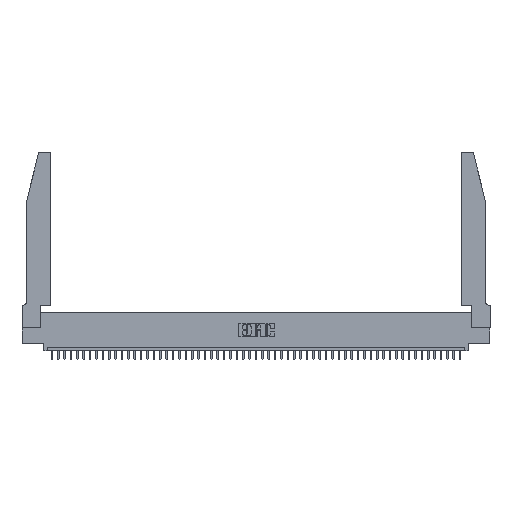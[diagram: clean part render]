
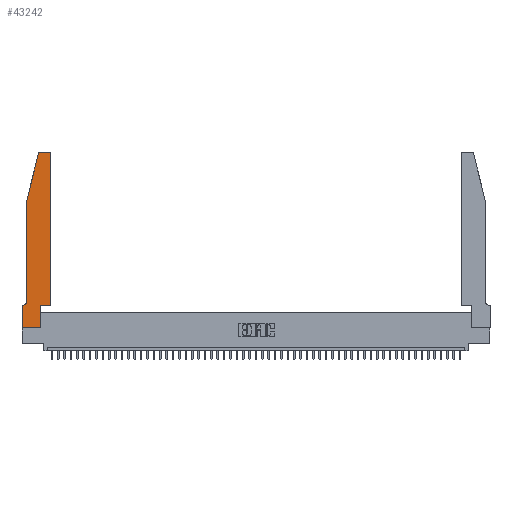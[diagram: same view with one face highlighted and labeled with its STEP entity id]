
A CAD part, top view. The second image highlights one B-rep face of the part: STEP entity #43242.
In plain terms, the highlighted planar face has unit normal (0, 0, 1).
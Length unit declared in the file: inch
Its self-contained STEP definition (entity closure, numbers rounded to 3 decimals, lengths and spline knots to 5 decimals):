
#495 = EDGE_CURVE ( 'NONE', #29341, #40950, #36946, .T. ) ;
#590 = EDGE_CURVE ( 'NONE', #809, #47112, #31429, .T. ) ;
#809 = VERTEX_POINT ( 'NONE', #6096 ) ;
#1147 = ORIENTED_EDGE ( 'NONE', *, *, #14008, .T. ) ;
#1455 = CARTESIAN_POINT ( 'NONE',  ( 0.0755, 0.35, 0.37 ) ) ;
#1528 = DIRECTION ( 'NONE',  ( -0.239, -0.971, 0. ) ) ;
#2582 = EDGE_CURVE ( 'NONE', #37422, #9412, #15421, .T. ) ;
#3336 = VERTEX_POINT ( 'NONE', #26846 ) ;
#4393 = CARTESIAN_POINT ( 'NONE',  ( 0.2865, 0.35, 0.37 ) ) ;
#5661 = CARTESIAN_POINT ( 'NONE',  ( 0.4205, 2.75, 0.37 ) ) ;
#5917 = CARTESIAN_POINT ( 'NONE',  ( 0.0055, 0.42, 0.37 ) ) ;
#6055 = DIRECTION ( 'NONE',  ( 0., 1., 0. ) ) ;
#6062 = LINE ( 'NONE', #7796, #25618 ) ;
#6096 = CARTESIAN_POINT ( 'NONE',  ( 0., 0., 0.37 ) ) ;
#7111 = EDGE_CURVE ( 'NONE', #3336, #15386, #10087, .T. ) ;
#7328 = ORIENTED_EDGE ( 'NONE', *, *, #14527, .T. ) ;
#7796 = CARTESIAN_POINT ( 'NONE',  ( 0.0755, 2., 0.37 ) ) ;
#8619 = ORIENTED_EDGE ( 'NONE', *, *, #26098, .T. ) ;
#8633 = PLANE ( 'NONE',  #12417 ) ;
#8872 = EDGE_CURVE ( 'NONE', #28863, #3336, #14033, .T. ) ;
#9007 = CARTESIAN_POINT ( 'NONE',  ( 0.4505, 0.35, 0.37 ) ) ;
#9250 = CIRCLE ( 'NONE', #36645, 0.03 ) ;
#9412 = VERTEX_POINT ( 'NONE', #22012 ) ;
#9848 = LINE ( 'NONE', #14392, #38137 ) ;
#9926 = VECTOR ( 'NONE', #36246, 39.37008 ) ;
#10087 = LINE ( 'NONE', #1455, #43846 ) ;
#11253 = DIRECTION ( 'NONE',  ( -1., 0., 0. ) ) ;
#11617 = DIRECTION ( 'NONE',  ( 1., 0., 0. ) ) ;
#11722 = VECTOR ( 'NONE', #1528, 39.37008 ) ;
#12343 = CIRCLE ( 'NONE', #21338, 0.03 ) ;
#12417 = AXIS2_PLACEMENT_3D ( 'NONE', #43455, #39219, #27490 ) ;
#13644 = EDGE_LOOP ( 'NONE', ( #7328, #49788, #37981, #8619, #37603, #48572, #25549, #42449, #34405, #46045, #41662, #1147 ) ) ;
#13886 = DIRECTION ( 'NONE',  ( 1., 0., 0. ) ) ;
#14008 = EDGE_CURVE ( 'NONE', #40950, #33710, #9250, .T. ) ;
#14033 = CIRCLE ( 'NONE', #16142, 0.07 ) ;
#14392 = CARTESIAN_POINT ( 'NONE',  ( 0.2865, 0.35, 0.37 ) ) ;
#14524 = DIRECTION ( 'NONE',  ( 0., -1., 0. ) ) ;
#14527 = EDGE_CURVE ( 'NONE', #33710, #45415, #20190, .T. ) ;
#15218 = CARTESIAN_POINT ( 'NONE',  ( 0.2605, 2.75, 0.37 ) ) ;
#15386 = VERTEX_POINT ( 'NONE', #41756 ) ;
#15421 = LINE ( 'NONE', #40391, #11722 ) ;
#16142 = AXIS2_PLACEMENT_3D ( 'NONE', #5917, #32952, #17025 ) ;
#17025 = DIRECTION ( 'NONE',  ( -1., 0., 0. ) ) ;
#18484 = CARTESIAN_POINT ( 'NONE',  ( 0., 0., 0.37 ) ) ;
#20190 = LINE ( 'NONE', #15218, #36044 ) ;
#20630 = DIRECTION ( 'NONE',  ( 0., 1., 0. ) ) ;
#20795 = CARTESIAN_POINT ( 'NONE',  ( 0.4505, 0.35, 0.37 ) ) ;
#21338 = AXIS2_PLACEMENT_3D ( 'NONE', #27720, #23126, #11617 ) ;
#22012 = CARTESIAN_POINT ( 'NONE',  ( 0.0755, 2., 0.37 ) ) ;
#22039 = DIRECTION ( 'NONE',  ( 1., 0., 0. ) ) ;
#23126 = DIRECTION ( 'NONE',  ( 0., 0., 1. ) ) ;
#24107 = VECTOR ( 'NONE', #14524, 39.37008 ) ;
#24660 = VECTOR ( 'NONE', #20630, 39.37008 ) ;
#25549 = ORIENTED_EDGE ( 'NONE', *, *, #44406, .T. ) ;
#25618 = VECTOR ( 'NONE', #35502, 39.37008 ) ;
#26098 = EDGE_CURVE ( 'NONE', #9412, #28863, #6062, .T. ) ;
#26796 = CARTESIAN_POINT ( 'NONE',  ( 0.4505, 2.72, 0.37 ) ) ;
#26846 = CARTESIAN_POINT ( 'NONE',  ( 0.0055, 0.35, 0.37 ) ) ;
#27490 = DIRECTION ( 'NONE',  ( 1., 0., 0. ) ) ;
#27720 = CARTESIAN_POINT ( 'NONE',  ( 0.284, 2.72, 0.37 ) ) ;
#28027 = EDGE_CURVE ( 'NONE', #47112, #39660, #9848, .T. ) ;
#28863 = VERTEX_POINT ( 'NONE', #43666 ) ;
#29341 = VERTEX_POINT ( 'NONE', #9007 ) ;
#31429 = LINE ( 'NONE', #32120, #9926 ) ;
#32120 = CARTESIAN_POINT ( 'NONE',  ( 0., 0., 0.37 ) ) ;
#32740 = DIRECTION ( 'NONE',  ( -1., 0., 0. ) ) ;
#32952 = DIRECTION ( 'NONE',  ( 0., 0., -1. ) ) ;
#33083 = DIRECTION ( 'NONE',  ( 0., 0., 1. ) ) ;
#33300 = CARTESIAN_POINT ( 'NONE',  ( 0.2865, 0., 0.37 ) ) ;
#33710 = VERTEX_POINT ( 'NONE', #5661 ) ;
#34405 = ORIENTED_EDGE ( 'NONE', *, *, #28027, .T. ) ;
#35502 = DIRECTION ( 'NONE',  ( 0., -1., 0. ) ) ;
#35896 = VECTOR ( 'NONE', #22039, 39.37008 ) ;
#36044 = VECTOR ( 'NONE', #11253, 39.37008 ) ;
#36246 = DIRECTION ( 'NONE',  ( 1., 0., 0. ) ) ;
#36645 = AXIS2_PLACEMENT_3D ( 'NONE', #37403, #33083, #13886 ) ;
#36946 = LINE ( 'NONE', #20795, #24660 ) ;
#37403 = CARTESIAN_POINT ( 'NONE',  ( 0.4205, 2.72, 0.37 ) ) ;
#37422 = VERTEX_POINT ( 'NONE', #47876 ) ;
#37603 = ORIENTED_EDGE ( 'NONE', *, *, #8872, .T. ) ;
#37885 = CARTESIAN_POINT ( 'NONE',  ( 0.4505, 0.35, 0.37 ) ) ;
#37981 = ORIENTED_EDGE ( 'NONE', *, *, #2582, .T. ) ;
#38137 = VECTOR ( 'NONE', #6055, 39.37008 ) ;
#39219 = DIRECTION ( 'NONE',  ( 0., 0., 1. ) ) ;
#39660 = VERTEX_POINT ( 'NONE', #4393 ) ;
#40391 = CARTESIAN_POINT ( 'NONE',  ( 0.0755, 2., 0.37 ) ) ;
#40950 = VERTEX_POINT ( 'NONE', #26796 ) ;
#41662 = ORIENTED_EDGE ( 'NONE', *, *, #495, .T. ) ;
#41756 = CARTESIAN_POINT ( 'NONE',  ( 0., 0.35, 0.37 ) ) ;
#42449 = ORIENTED_EDGE ( 'NONE', *, *, #590, .T. ) ;
#43242 = ADVANCED_FACE ( 'NONE', ( #45100 ), #8633, .T. ) ;
#43455 = CARTESIAN_POINT ( 'NONE',  ( 0., 0.35, 0.37 ) ) ;
#43666 = CARTESIAN_POINT ( 'NONE',  ( 0.0755, 0.42, 0.37 ) ) ;
#43778 = LINE ( 'NONE', #18484, #24107 ) ;
#43846 = VECTOR ( 'NONE', #32740, 39.37008 ) ;
#44406 = EDGE_CURVE ( 'NONE', #15386, #809, #43778, .T. ) ;
#45100 = FACE_OUTER_BOUND ( 'NONE', #13644, .T. ) ;
#45415 = VERTEX_POINT ( 'NONE', #49779 ) ;
#46045 = ORIENTED_EDGE ( 'NONE', *, *, #50469, .T. ) ;
#46108 = EDGE_CURVE ( 'NONE', #45415, #37422, #12343, .T. ) ;
#47112 = VERTEX_POINT ( 'NONE', #33300 ) ;
#47876 = CARTESIAN_POINT ( 'NONE',  ( 0.25487, 2.72718, 0.37 ) ) ;
#48572 = ORIENTED_EDGE ( 'NONE', *, *, #7111, .T. ) ;
#49779 = CARTESIAN_POINT ( 'NONE',  ( 0.284, 2.75, 0.37 ) ) ;
#49788 = ORIENTED_EDGE ( 'NONE', *, *, #46108, .T. ) ;
#50036 = LINE ( 'NONE', #37885, #35896 ) ;
#50469 = EDGE_CURVE ( 'NONE', #39660, #29341, #50036, .T. ) ;
